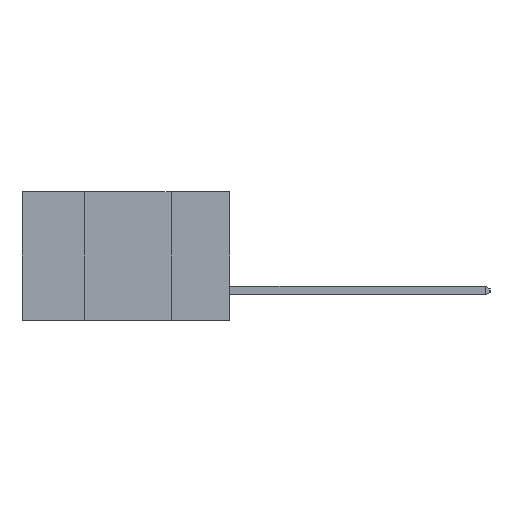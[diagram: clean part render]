
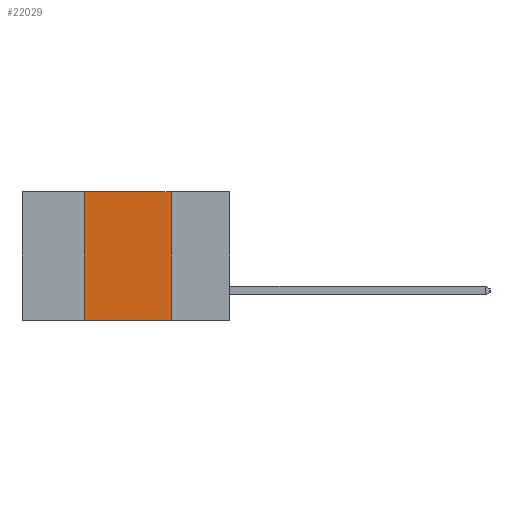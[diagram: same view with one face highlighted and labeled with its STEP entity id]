
A CAD part, left-side view. The second image highlights one B-rep face of the part: STEP entity #22029.
In plain terms, the highlighted planar face has unit normal (-1, 0, 0).
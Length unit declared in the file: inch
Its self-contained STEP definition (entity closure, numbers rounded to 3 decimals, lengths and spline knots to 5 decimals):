
#291 = FACE_OUTER_BOUND ( 'NONE', #22378, .T. ) ;
#340 = DIRECTION ( 'NONE',  ( 0., -1., 0. ) ) ;
#567 = CARTESIAN_POINT ( 'NONE',  ( 0., 0.17, -0.37 ) ) ;
#3282 = VERTEX_POINT ( 'NONE', #567 ) ;
#3759 = CARTESIAN_POINT ( 'NONE',  ( 0., 0.6, 0. ) ) ;
#3843 = LINE ( 'NONE', #11708, #20188 ) ;
#5244 = DIRECTION ( 'NONE',  ( 0., -1., 0. ) ) ;
#5492 = ORIENTED_EDGE ( 'NONE', *, *, #22318, .F. ) ;
#6999 = CARTESIAN_POINT ( 'NONE',  ( 0., 0.42, 0. ) ) ;
#7104 = LINE ( 'NONE', #9749, #11416 ) ;
#7902 = EDGE_CURVE ( 'NONE', #20071, #3282, #25658, .T. ) ;
#8234 = CARTESIAN_POINT ( 'NONE',  ( 0., 0.17, 0. ) ) ;
#8240 = PLANE ( 'NONE',  #10472 ) ;
#9089 = DIRECTION ( 'NONE',  ( 0., 0., -1. ) ) ;
#9697 = CARTESIAN_POINT ( 'NONE',  ( 0., 0.42, -0.37 ) ) ;
#9749 = CARTESIAN_POINT ( 'NONE',  ( 0., 0.6, -0.37 ) ) ;
#10472 = AXIS2_PLACEMENT_3D ( 'NONE', #3759, #10643, #25856 ) ;
#10643 = DIRECTION ( 'NONE',  ( 1., 0., 0. ) ) ;
#11416 = VECTOR ( 'NONE', #5244, 39.37008 ) ;
#11708 = CARTESIAN_POINT ( 'NONE',  ( 0., 0.6, 0. ) ) ;
#11894 = ORIENTED_EDGE ( 'NONE', *, *, #7902, .F. ) ;
#12704 = EDGE_CURVE ( 'NONE', #24863, #3282, #7104, .T. ) ;
#13178 = LINE ( 'NONE', #23049, #24661 ) ;
#14127 = VECTOR ( 'NONE', #9089, 39.37008 ) ;
#16646 = DIRECTION ( 'NONE',  ( 0., 0., 1. ) ) ;
#16844 = EDGE_CURVE ( 'NONE', #24863, #21026, #13178, .T. ) ;
#19710 = ORIENTED_EDGE ( 'NONE', *, *, #12704, .T. ) ;
#20036 = CARTESIAN_POINT ( 'NONE',  ( 0., 0.17, 0. ) ) ;
#20071 = VERTEX_POINT ( 'NONE', #8234 ) ;
#20188 = VECTOR ( 'NONE', #340, 39.37008 ) ;
#21026 = VERTEX_POINT ( 'NONE', #6999 ) ;
#22029 = ADVANCED_FACE ( 'NONE', ( #291 ), #8240, .F. ) ;
#22318 = EDGE_CURVE ( 'NONE', #21026, #20071, #3843, .T. ) ;
#22378 = EDGE_LOOP ( 'NONE', ( #11894, #5492, #25123, #19710 ) ) ;
#23049 = CARTESIAN_POINT ( 'NONE',  ( 0., 0.42, 0. ) ) ;
#24661 = VECTOR ( 'NONE', #16646, 39.37008 ) ;
#24863 = VERTEX_POINT ( 'NONE', #9697 ) ;
#25123 = ORIENTED_EDGE ( 'NONE', *, *, #16844, .F. ) ;
#25658 = LINE ( 'NONE', #20036, #14127 ) ;
#25856 = DIRECTION ( 'NONE',  ( 0., 0., -1. ) ) ;
